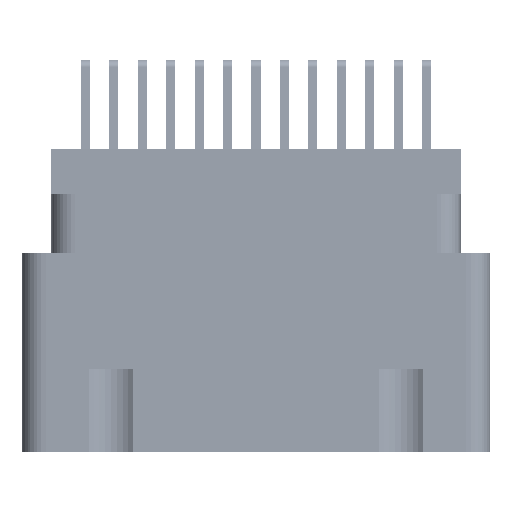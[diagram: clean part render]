
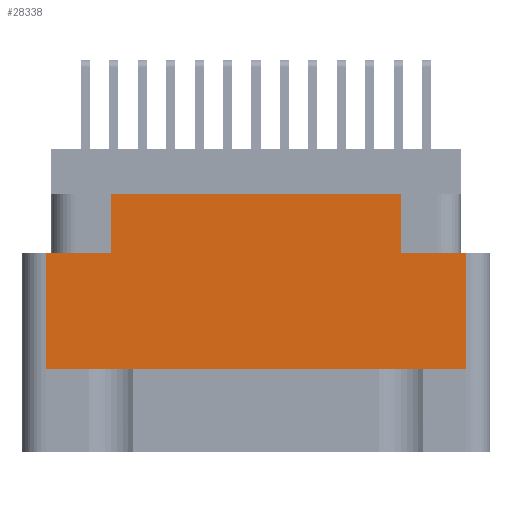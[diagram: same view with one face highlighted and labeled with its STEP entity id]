
A CAD part, left-side view. The second image highlights one B-rep face of the part: STEP entity #28338.
In plain terms, the highlighted planar face has unit normal (-1, 0, 0).
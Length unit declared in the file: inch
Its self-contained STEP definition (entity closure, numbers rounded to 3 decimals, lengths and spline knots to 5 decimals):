
#390 = FACE_OUTER_BOUND ( 'NONE', #19569, .T. ) ;
#718 = DIRECTION ( 'NONE',  ( -1., 0., 0. ) ) ;
#1017 = DIRECTION ( 'NONE',  ( 0., -1., 0. ) ) ;
#2449 = ORIENTED_EDGE ( 'NONE', *, *, #9104, .T. ) ;
#5248 = AXIS2_PLACEMENT_3D ( 'NONE', #16187, #718, #21674 ) ;
#5992 = ORIENTED_EDGE ( 'NONE', *, *, #50068, .T. ) ;
#6284 = LINE ( 'NONE', #21413, #61040 ) ;
#6556 = EDGE_CURVE ( 'NONE', #7970, #54126, #26285, .T. ) ;
#7040 = ORIENTED_EDGE ( 'NONE', *, *, #23752, .T. ) ;
#7970 = VERTEX_POINT ( 'NONE', #39987 ) ;
#8474 = LINE ( 'NONE', #55562, #10207 ) ;
#9104 = EDGE_CURVE ( 'NONE', #59191, #29081, #6284, .T. ) ;
#9181 = LINE ( 'NONE', #18806, #66280 ) ;
#10207 = VECTOR ( 'NONE', #62054, 39.37008 ) ;
#11644 = CARTESIAN_POINT ( 'NONE',  ( -1.359, 0.3825, -0.117 ) ) ;
#15208 = VECTOR ( 'NONE', #41027, 39.37008 ) ;
#16187 = CARTESIAN_POINT ( 'NONE',  ( -1.359, -0.617, -0.798 ) ) ;
#16457 = LINE ( 'NONE', #62549, #33288 ) ;
#16651 = DIRECTION ( 'NONE',  ( 0., 0., 1. ) ) ;
#17517 = CARTESIAN_POINT ( 'NONE',  ( -1.359, 0.555, -0.274 ) ) ;
#18806 = CARTESIAN_POINT ( 'NONE',  ( -1.359, 0., -0.274 ) ) ;
#19241 = DIRECTION ( 'NONE',  ( 0., 0., 1. ) ) ;
#19569 = EDGE_LOOP ( 'NONE', ( #32030, #2449, #7040, #40964, #28880, #5992, #46678, #20805 ) ) ;
#20529 = VERTEX_POINT ( 'NONE', #31477 ) ;
#20805 = ORIENTED_EDGE ( 'NONE', *, *, #32684, .F. ) ;
#21413 = CARTESIAN_POINT ( 'NONE',  ( -1.359, 0.555, -0.798 ) ) ;
#21674 = DIRECTION ( 'NONE',  ( 0., 0., 1. ) ) ;
#23752 = EDGE_CURVE ( 'NONE', #29081, #7970, #16457, .T. ) ;
#23795 = VECTOR ( 'NONE', #19241, 39.37008 ) ;
#23839 = VERTEX_POINT ( 'NONE', #11644 ) ;
#26285 = LINE ( 'NONE', #43089, #58709 ) ;
#28338 = ADVANCED_FACE ( 'NONE', ( #390 ), #47794, .T. ) ;
#28880 = ORIENTED_EDGE ( 'NONE', *, *, #47678, .F. ) ;
#29081 = VERTEX_POINT ( 'NONE', #60243 ) ;
#30906 = LINE ( 'NONE', #40874, #23795 ) ;
#31477 = CARTESIAN_POINT ( 'NONE',  ( -1.359, -0.3825, -0.274 ) ) ;
#31939 = CARTESIAN_POINT ( 'NONE',  ( -1.359, 0., -0.274 ) ) ;
#32030 = ORIENTED_EDGE ( 'NONE', *, *, #61009, .F. ) ;
#32684 = EDGE_CURVE ( 'NONE', #49577, #23839, #30906, .T. ) ;
#33288 = VECTOR ( 'NONE', #52898, 39.37008 ) ;
#39987 = CARTESIAN_POINT ( 'NONE',  ( -1.359, -0.555, -0.578 ) ) ;
#40580 = EDGE_CURVE ( 'NONE', #23839, #47835, #8474, .T. ) ;
#40874 = CARTESIAN_POINT ( 'NONE',  ( -1.359, 0.3825, -0.274 ) ) ;
#40964 = ORIENTED_EDGE ( 'NONE', *, *, #6556, .T. ) ;
#41027 = DIRECTION ( 'NONE',  ( 0., 0., 1. ) ) ;
#43089 = CARTESIAN_POINT ( 'NONE',  ( -1.359, -0.555, -0.798 ) ) ;
#46678 = ORIENTED_EDGE ( 'NONE', *, *, #40580, .F. ) ;
#47678 = EDGE_CURVE ( 'NONE', #20529, #54126, #58422, .T. ) ;
#47794 = PLANE ( 'NONE',  #5248 ) ;
#47835 = VERTEX_POINT ( 'NONE', #49119 ) ;
#47957 = CARTESIAN_POINT ( 'NONE',  ( -1.359, 0.3825, -0.274 ) ) ;
#49119 = CARTESIAN_POINT ( 'NONE',  ( -1.359, -0.3825, -0.117 ) ) ;
#49577 = VERTEX_POINT ( 'NONE', #47957 ) ;
#50068 = EDGE_CURVE ( 'NONE', #20529, #47835, #67178, .T. ) ;
#52898 = DIRECTION ( 'NONE',  ( 0., -1., 0. ) ) ;
#54126 = VERTEX_POINT ( 'NONE', #56334 ) ;
#55562 = CARTESIAN_POINT ( 'NONE',  ( -1.359, 0.617, -0.117 ) ) ;
#56334 = CARTESIAN_POINT ( 'NONE',  ( -1.359, -0.555, -0.274 ) ) ;
#58203 = CARTESIAN_POINT ( 'NONE',  ( -1.359, -0.3825, -0.274 ) ) ;
#58422 = LINE ( 'NONE', #31939, #65655 ) ;
#58709 = VECTOR ( 'NONE', #16651, 39.37008 ) ;
#59191 = VERTEX_POINT ( 'NONE', #17517 ) ;
#60243 = CARTESIAN_POINT ( 'NONE',  ( -1.359, 0.555, -0.578 ) ) ;
#61009 = EDGE_CURVE ( 'NONE', #59191, #49577, #9181, .T. ) ;
#61040 = VECTOR ( 'NONE', #67860, 39.37008 ) ;
#62054 = DIRECTION ( 'NONE',  ( 0., -1., 0. ) ) ;
#62549 = CARTESIAN_POINT ( 'NONE',  ( -1.359, 0., -0.578 ) ) ;
#65655 = VECTOR ( 'NONE', #1017, 39.37008 ) ;
#66254 = DIRECTION ( 'NONE',  ( 0., -1., 0. ) ) ;
#66280 = VECTOR ( 'NONE', #66254, 39.37008 ) ;
#67178 = LINE ( 'NONE', #58203, #15208 ) ;
#67860 = DIRECTION ( 'NONE',  ( 0., 0., -1. ) ) ;
